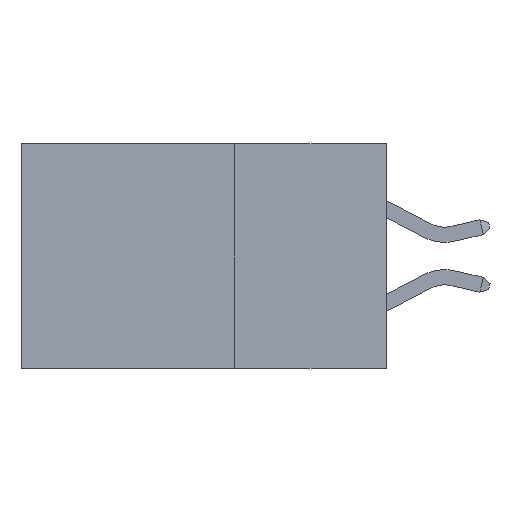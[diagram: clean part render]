
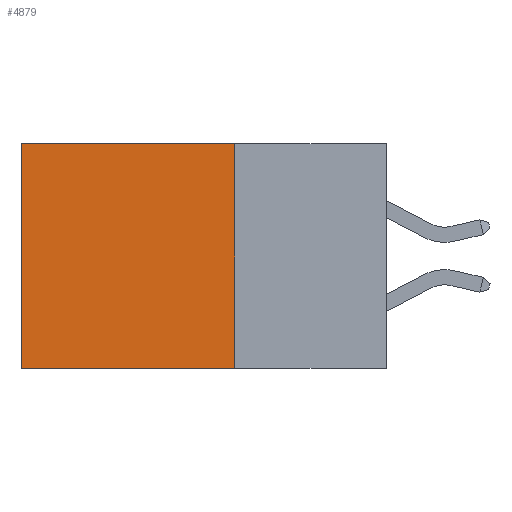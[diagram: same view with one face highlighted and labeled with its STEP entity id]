
A CAD part, left-side view. The second image highlights one B-rep face of the part: STEP entity #4879.
In plain terms, the highlighted planar face has unit normal (-1, 0, 0).
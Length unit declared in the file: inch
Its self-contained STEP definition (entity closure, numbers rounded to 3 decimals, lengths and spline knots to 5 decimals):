
#46 = LINE ( 'NONE', #4711, #8761 ) ;
#267 = DIRECTION ( 'NONE',  ( 0., 0., -1. ) ) ;
#495 = CARTESIAN_POINT ( 'NONE',  ( 0.2615, 0.6, -0.37 ) ) ;
#793 = LINE ( 'NONE', #495, #1545 ) ;
#895 = EDGE_CURVE ( 'NONE', #5777, #6955, #1408, .T. ) ;
#1174 = CARTESIAN_POINT ( 'NONE',  ( 0.2615, 0.25, 0. ) ) ;
#1282 = DIRECTION ( 'NONE',  ( 0., 1., 0. ) ) ;
#1284 = EDGE_CURVE ( 'NONE', #9050, #4953, #46, .T. ) ;
#1408 = LINE ( 'NONE', #1174, #1662 ) ;
#1545 = VECTOR ( 'NONE', #6799, 39.37008 ) ;
#1662 = VECTOR ( 'NONE', #1282, 39.37008 ) ;
#2116 = DIRECTION ( 'NONE',  ( 0., 0., -1. ) ) ;
#2180 = FACE_OUTER_BOUND ( 'NONE', #9683, .T. ) ;
#2596 = PLANE ( 'NONE',  #8585 ) ;
#2989 = CARTESIAN_POINT ( 'NONE',  ( 0.2615, 0.25, -0.37 ) ) ;
#3417 = ORIENTED_EDGE ( 'NONE', *, *, #1284, .F. ) ;
#3848 = LINE ( 'NONE', #6899, #6925 ) ;
#4711 = CARTESIAN_POINT ( 'NONE',  ( 0.2615, 0.25, -0.37 ) ) ;
#4879 = ADVANCED_FACE ( 'NONE', ( #2180 ), #2596, .F. ) ;
#4953 = VERTEX_POINT ( 'NONE', #6797 ) ;
#5000 = CARTESIAN_POINT ( 'NONE',  ( 0.2615, 0.6, 0. ) ) ;
#5777 = VERTEX_POINT ( 'NONE', #6208 ) ;
#6208 = CARTESIAN_POINT ( 'NONE',  ( 0.2615, 0.25, 0. ) ) ;
#6227 = EDGE_CURVE ( 'NONE', #6955, #4953, #793, .T. ) ;
#6797 = CARTESIAN_POINT ( 'NONE',  ( 0.2615, 0.6, -0.37 ) ) ;
#6799 = DIRECTION ( 'NONE',  ( 0., 0., -1. ) ) ;
#6899 = CARTESIAN_POINT ( 'NONE',  ( 0.2615, 0.25, -0.37 ) ) ;
#6925 = VECTOR ( 'NONE', #2116, 39.37008 ) ;
#6955 = VERTEX_POINT ( 'NONE', #5000 ) ;
#7340 = DIRECTION ( 'NONE',  ( 1., 0., 0. ) ) ;
#7512 = EDGE_CURVE ( 'NONE', #5777, #9050, #3848, .T. ) ;
#8096 = ORIENTED_EDGE ( 'NONE', *, *, #895, .T. ) ;
#8310 = ORIENTED_EDGE ( 'NONE', *, *, #6227, .T. ) ;
#8585 = AXIS2_PLACEMENT_3D ( 'NONE', #8984, #7340, #267 ) ;
#8742 = DIRECTION ( 'NONE',  ( 0., 1., 0. ) ) ;
#8761 = VECTOR ( 'NONE', #8742, 39.37008 ) ;
#8984 = CARTESIAN_POINT ( 'NONE',  ( 0.2615, 0.25, -0.37 ) ) ;
#9050 = VERTEX_POINT ( 'NONE', #2989 ) ;
#9446 = ORIENTED_EDGE ( 'NONE', *, *, #7512, .F. ) ;
#9683 = EDGE_LOOP ( 'NONE', ( #8310, #3417, #9446, #8096 ) ) ;
